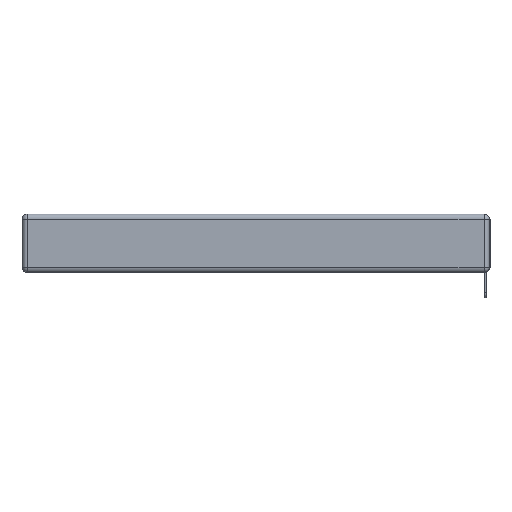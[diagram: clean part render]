
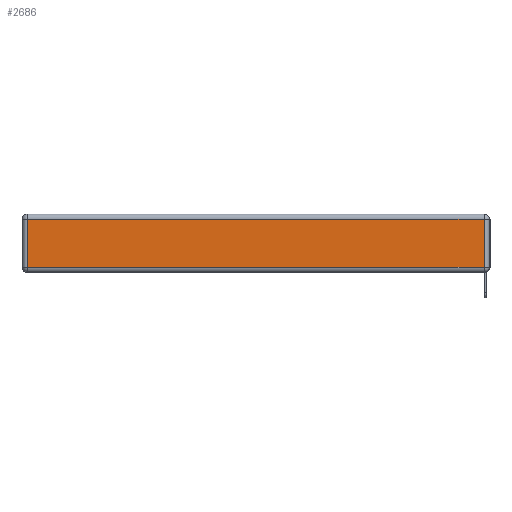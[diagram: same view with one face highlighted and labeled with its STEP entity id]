
A CAD part, left-side view. The second image highlights one B-rep face of the part: STEP entity #2686.
In plain terms, the highlighted planar face has unit normal (-1, 0, 0).
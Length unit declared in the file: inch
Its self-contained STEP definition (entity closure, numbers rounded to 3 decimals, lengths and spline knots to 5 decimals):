
#201 = EDGE_CURVE ( 'NONE', #12525, #8599, #11259, .T. ) ;
#250 = DIRECTION ( 'NONE',  ( 0., 0., -1. ) ) ;
#477 = CARTESIAN_POINT ( 'NONE',  ( 0., 2.72, -0.343 ) ) ;
#902 = CARTESIAN_POINT ( 'NONE',  ( 0., 0., -0.343 ) ) ;
#983 = DIRECTION ( 'NONE',  ( -1., 0., 0. ) ) ;
#1231 = VECTOR ( 'NONE', #6132, 39.37008 ) ;
#1439 = VECTOR ( 'NONE', #250, 39.37008 ) ;
#1666 = EDGE_CURVE ( 'NONE', #7579, #4687, #1787, .T. ) ;
#1709 = CARTESIAN_POINT ( 'NONE',  ( 0., 0.03, -0.343 ) ) ;
#1787 = LINE ( 'NONE', #1709, #7812 ) ;
#2265 = CARTESIAN_POINT ( 'NONE',  ( 0., 2.75, -0.03 ) ) ;
#2329 = FACE_OUTER_BOUND ( 'NONE', #3306, .T. ) ;
#2409 = PLANE ( 'NONE',  #3152 ) ;
#2686 = ADVANCED_FACE ( 'NONE', ( #2329 ), #2409, .T. ) ;
#3152 = AXIS2_PLACEMENT_3D ( 'NONE', #902, #983, #7144 ) ;
#3306 = EDGE_LOOP ( 'NONE', ( #13369, #11100, #9352, #9434 ) ) ;
#4122 = CARTESIAN_POINT ( 'NONE',  ( 0., 2.72, -0.03 ) ) ;
#4687 = VERTEX_POINT ( 'NONE', #10087 ) ;
#4798 = LINE ( 'NONE', #2265, #1231 ) ;
#5483 = CARTESIAN_POINT ( 'NONE',  ( 0., 2.72, -0.313 ) ) ;
#5861 = VECTOR ( 'NONE', #14629, 39.37008 ) ;
#6132 = DIRECTION ( 'NONE',  ( 0., 1., 0. ) ) ;
#6591 = DIRECTION ( 'NONE',  ( 0., 0., 1. ) ) ;
#6627 = EDGE_CURVE ( 'NONE', #4687, #12525, #4798, .T. ) ;
#7144 = DIRECTION ( 'NONE',  ( 0., 0., 1. ) ) ;
#7579 = VERTEX_POINT ( 'NONE', #7789 ) ;
#7789 = CARTESIAN_POINT ( 'NONE',  ( 0., 0.03, -0.313 ) ) ;
#7812 = VECTOR ( 'NONE', #6591, 39.37008 ) ;
#8599 = VERTEX_POINT ( 'NONE', #5483 ) ;
#9352 = ORIENTED_EDGE ( 'NONE', *, *, #6627, .T. ) ;
#9434 = ORIENTED_EDGE ( 'NONE', *, *, #201, .T. ) ;
#10087 = CARTESIAN_POINT ( 'NONE',  ( 0., 0.03, -0.03 ) ) ;
#10096 = LINE ( 'NONE', #14854, #5861 ) ;
#11100 = ORIENTED_EDGE ( 'NONE', *, *, #1666, .T. ) ;
#11259 = LINE ( 'NONE', #477, #1439 ) ;
#12045 = EDGE_CURVE ( 'NONE', #8599, #7579, #10096, .T. ) ;
#12525 = VERTEX_POINT ( 'NONE', #4122 ) ;
#13369 = ORIENTED_EDGE ( 'NONE', *, *, #12045, .T. ) ;
#14629 = DIRECTION ( 'NONE',  ( 0., -1., 0. ) ) ;
#14854 = CARTESIAN_POINT ( 'NONE',  ( 0., 0., -0.313 ) ) ;
